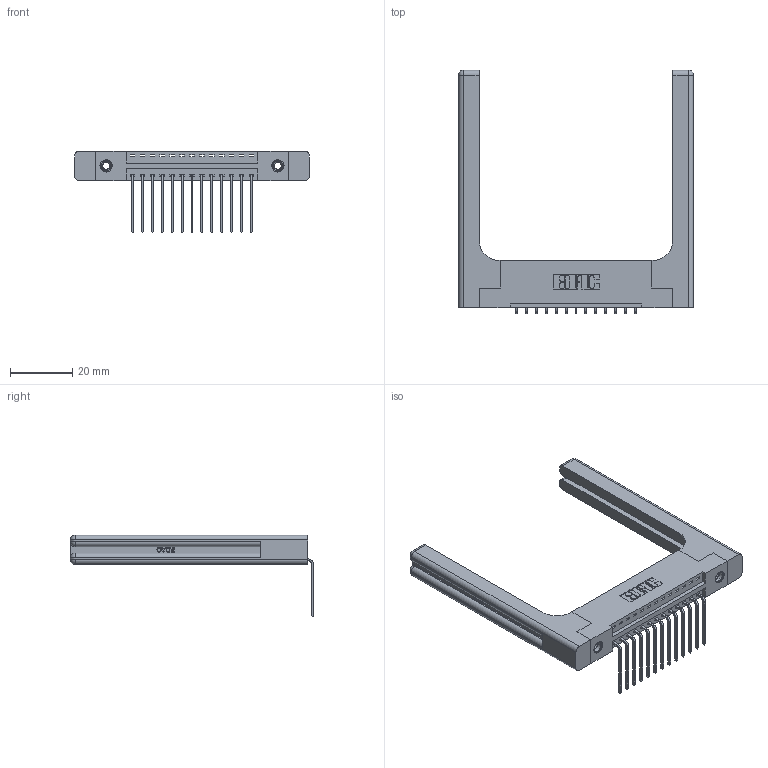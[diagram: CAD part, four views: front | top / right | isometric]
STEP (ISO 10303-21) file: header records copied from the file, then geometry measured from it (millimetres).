
FILE_DESCRIPTION (( 'STEP AP203' ), '1' );
FILE_NAME ('346-013-559-158.STEP', '2022-05-05T05:19:24', ( '' ), ( '' ), 'SwSTEP 2.0', 'SolidWorks 2020', '' );
FILE_SCHEMA (( 'CONFIG_CONTROL_DESIGN' ));
Length unit declared in the file: inch
Products named in the file (5): 345-292-001_558 559 Tail - 1; 345-250-001_345-250-001-102; 346 Part_Flush Mounting Lugs - 0.156 Dia-TH; 346-220-058_345-220-058; 346-013-559-158
Assembly tree (18 placements, depth 2):
  346-013-559-158
    346 Part_Flush Mounting Lugs - 0.156 Dia-TH
    345-292-001_558 559 Tail - 1  x13
    345-250-001_345-250-001-102  x2
    346-220-058_345-220-058  x2
Bounding box: 75.34 x 78.04 x 26.16 mm (x, y, z)
Volume: 14555.2 mm3; surface area: 13942.3 mm2
Topology: 18 solids, 18 shells, 1172 faces, 3397 edges, 2226 vertices
Faces by surface type: plane 784, cylinder 328, bspline 36, cone 12, sphere 8, torus 4
Entity records: 17654 total; most frequent: CARTESIAN_POINT 4018, ORIENTED_EDGE 2760, DIRECTION 2510, EDGE_CURVE 1380, LINE 1104, VECTOR 1104, VERTEX_POINT 910, AXIS2_PLACEMENT_3D 703
